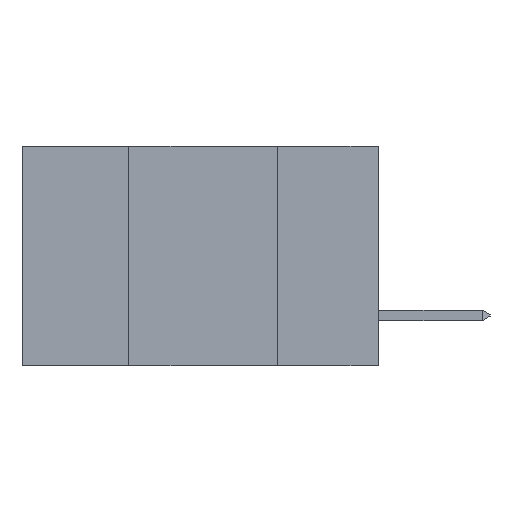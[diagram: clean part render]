
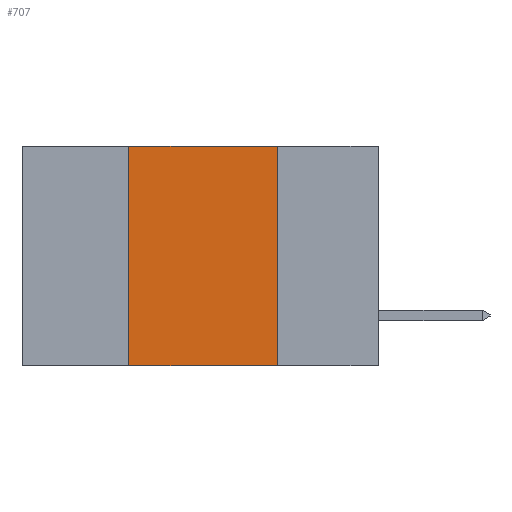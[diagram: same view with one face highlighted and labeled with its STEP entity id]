
A CAD part, left-side view. The second image highlights one B-rep face of the part: STEP entity #707.
In plain terms, the highlighted planar face has unit normal (-1, 0, 0).
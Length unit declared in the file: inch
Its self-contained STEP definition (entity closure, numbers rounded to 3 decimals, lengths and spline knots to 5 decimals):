
#52 = CARTESIAN_POINT ( 'NONE',  ( 0., 0.42, -0.37 ) ) ;
#660 = AXIS2_PLACEMENT_3D ( 'NONE', #10476, #10316, #10305 ) ;
#677 = VERTEX_POINT ( 'NONE', #11471 ) ;
#707 = ADVANCED_FACE ( 'NONE', ( #1164 ), #10531, .F. ) ;
#1164 = FACE_OUTER_BOUND ( 'NONE', #11962, .T. ) ;
#1926 = EDGE_CURVE ( 'NONE', #5277, #5334, #11761, .T. ) ;
#2343 = VECTOR ( 'NONE', #6388, 39.37008 ) ;
#2425 = LINE ( 'NONE', #10296, #7773 ) ;
#3082 = DIRECTION ( 'NONE',  ( 0., -1., 0. ) ) ;
#3184 = CARTESIAN_POINT ( 'NONE',  ( 0., 0.6, -0.37 ) ) ;
#3493 = CARTESIAN_POINT ( 'NONE',  ( 0., 0.17, -0.37 ) ) ;
#3850 = LINE ( 'NONE', #8339, #6907 ) ;
#5277 = VERTEX_POINT ( 'NONE', #52 ) ;
#5334 = VERTEX_POINT ( 'NONE', #3493 ) ;
#5513 = EDGE_CURVE ( 'NONE', #677, #7797, #3850, .T. ) ;
#5766 = VECTOR ( 'NONE', #3082, 39.37008 ) ;
#6151 = ORIENTED_EDGE ( 'NONE', *, *, #1926, .T. ) ;
#6180 = ORIENTED_EDGE ( 'NONE', *, *, #14086, .F. ) ;
#6388 = DIRECTION ( 'NONE',  ( 0., 0., 1. ) ) ;
#6907 = VECTOR ( 'NONE', #9523, 39.37008 ) ;
#7773 = VECTOR ( 'NONE', #8014, 39.37008 ) ;
#7797 = VERTEX_POINT ( 'NONE', #9979 ) ;
#8014 = DIRECTION ( 'NONE',  ( 0., 0., -1. ) ) ;
#8339 = CARTESIAN_POINT ( 'NONE',  ( 0., 0.6, 0. ) ) ;
#9523 = DIRECTION ( 'NONE',  ( 0., -1., 0. ) ) ;
#9938 = ORIENTED_EDGE ( 'NONE', *, *, #5513, .F. ) ;
#9979 = CARTESIAN_POINT ( 'NONE',  ( 0., 0.17, 0. ) ) ;
#10296 = CARTESIAN_POINT ( 'NONE',  ( 0., 0.17, -0.37 ) ) ;
#10305 = DIRECTION ( 'NONE',  ( 0., 0., -1. ) ) ;
#10316 = DIRECTION ( 'NONE',  ( 1., 0., 0. ) ) ;
#10476 = CARTESIAN_POINT ( 'NONE',  ( 0., 0.6, 0. ) ) ;
#10531 = PLANE ( 'NONE',  #660 ) ;
#11313 = EDGE_CURVE ( 'NONE', #5277, #677, #11385, .T. ) ;
#11385 = LINE ( 'NONE', #14219, #2343 ) ;
#11471 = CARTESIAN_POINT ( 'NONE',  ( 0., 0.42, 0. ) ) ;
#11761 = LINE ( 'NONE', #3184, #5766 ) ;
#11962 = EDGE_LOOP ( 'NONE', ( #6180, #9938, #12755, #6151 ) ) ;
#12755 = ORIENTED_EDGE ( 'NONE', *, *, #11313, .F. ) ;
#14086 = EDGE_CURVE ( 'NONE', #7797, #5334, #2425, .T. ) ;
#14219 = CARTESIAN_POINT ( 'NONE',  ( 0., 0.42, -0.37 ) ) ;
